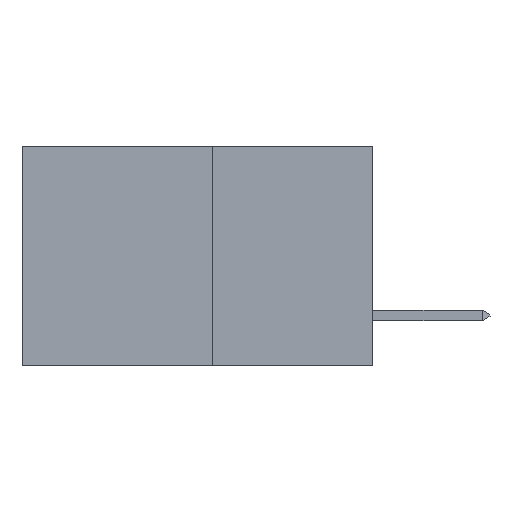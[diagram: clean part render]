
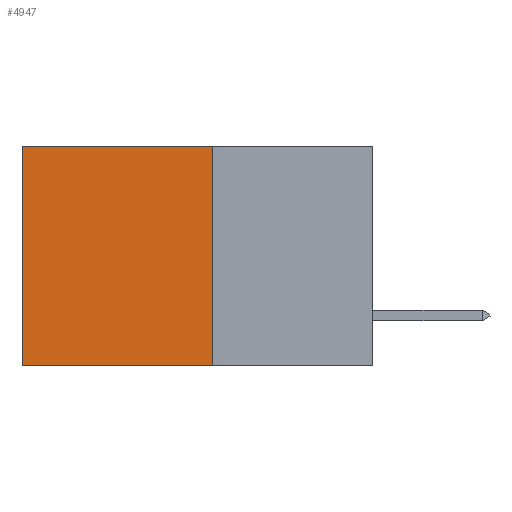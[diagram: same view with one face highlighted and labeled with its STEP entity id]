
A CAD part, left-side view. The second image highlights one B-rep face of the part: STEP entity #4947.
In plain terms, the highlighted planar face has unit normal (-1, 0, 0).
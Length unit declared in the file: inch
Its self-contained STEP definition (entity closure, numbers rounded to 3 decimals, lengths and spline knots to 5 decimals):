
#179 = VERTEX_POINT ( 'NONE', #2453 ) ;
#277 = AXIS2_PLACEMENT_3D ( 'NONE', #5941, #1231, #6770 ) ;
#463 = LINE ( 'NONE', #7150, #2553 ) ;
#546 = CARTESIAN_POINT ( 'NONE',  ( 0.277, 0.59, 0. ) ) ;
#601 = ORIENTED_EDGE ( 'NONE', *, *, #1990, .F. ) ;
#1163 = ORIENTED_EDGE ( 'NONE', *, *, #7024, .F. ) ;
#1231 = DIRECTION ( 'NONE',  ( 1., 0., 0. ) ) ;
#1352 = LINE ( 'NONE', #6807, #9304 ) ;
#1822 = ORIENTED_EDGE ( 'NONE', *, *, #4994, .T. ) ;
#1906 = CARTESIAN_POINT ( 'NONE',  ( 0.277, 0.27, 0. ) ) ;
#1990 = EDGE_CURVE ( 'NONE', #8652, #8814, #4567, .T. ) ;
#2114 = CARTESIAN_POINT ( 'NONE',  ( 0.277, 0.27, -0.37 ) ) ;
#2341 = CARTESIAN_POINT ( 'NONE',  ( 0.277, 0.27, -0.37 ) ) ;
#2453 = CARTESIAN_POINT ( 'NONE',  ( 0.277, 0.59, -0.37 ) ) ;
#2553 = VECTOR ( 'NONE', #3192, 39.37008 ) ;
#2904 = ORIENTED_EDGE ( 'NONE', *, *, #9042, .T. ) ;
#3192 = DIRECTION ( 'NONE',  ( 0., 0., -1. ) ) ;
#3464 = VECTOR ( 'NONE', #9471, 39.37008 ) ;
#3506 = VERTEX_POINT ( 'NONE', #546 ) ;
#3632 = CARTESIAN_POINT ( 'NONE',  ( 0.277, 0.27, -0.37 ) ) ;
#4567 = LINE ( 'NONE', #3632, #8590 ) ;
#4947 = ADVANCED_FACE ( 'NONE', ( #7684 ), #7552, .F. ) ;
#4994 = EDGE_CURVE ( 'NONE', #8652, #3506, #1352, .T. ) ;
#5211 = DIRECTION ( 'NONE',  ( 0., 1., 0. ) ) ;
#5330 = EDGE_LOOP ( 'NONE', ( #2904, #1163, #601, #1822 ) ) ;
#5941 = CARTESIAN_POINT ( 'NONE',  ( 0.277, 0.27, -0.37 ) ) ;
#6770 = DIRECTION ( 'NONE',  ( 0., 0., -1. ) ) ;
#6807 = CARTESIAN_POINT ( 'NONE',  ( 0.277, 0.27, 0. ) ) ;
#7024 = EDGE_CURVE ( 'NONE', #8814, #179, #7700, .T. ) ;
#7150 = CARTESIAN_POINT ( 'NONE',  ( 0.277, 0.59, -0.37 ) ) ;
#7469 = DIRECTION ( 'NONE',  ( 0., 0., -1. ) ) ;
#7552 = PLANE ( 'NONE',  #277 ) ;
#7684 = FACE_OUTER_BOUND ( 'NONE', #5330, .T. ) ;
#7700 = LINE ( 'NONE', #2341, #3464 ) ;
#8590 = VECTOR ( 'NONE', #7469, 39.37008 ) ;
#8652 = VERTEX_POINT ( 'NONE', #1906 ) ;
#8814 = VERTEX_POINT ( 'NONE', #2114 ) ;
#9042 = EDGE_CURVE ( 'NONE', #3506, #179, #463, .T. ) ;
#9304 = VECTOR ( 'NONE', #5211, 39.37008 ) ;
#9471 = DIRECTION ( 'NONE',  ( 0., 1., 0. ) ) ;
